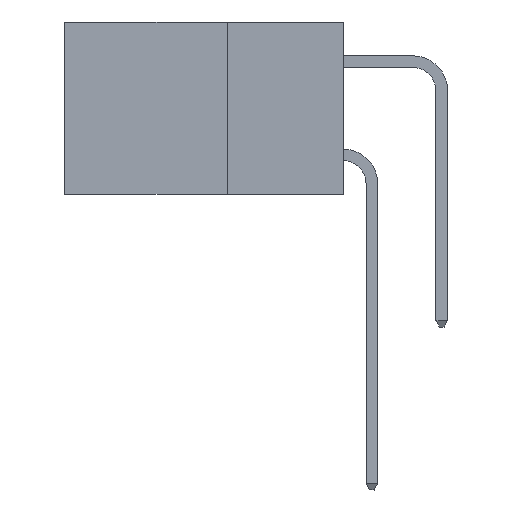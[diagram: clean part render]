
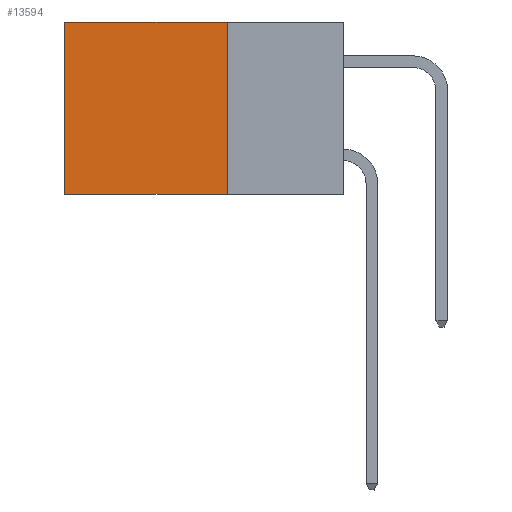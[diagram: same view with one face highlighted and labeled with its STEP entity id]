
A CAD part, left-side view. The second image highlights one B-rep face of the part: STEP entity #13594.
In plain terms, the highlighted planar face has unit normal (-1, 0, 0).
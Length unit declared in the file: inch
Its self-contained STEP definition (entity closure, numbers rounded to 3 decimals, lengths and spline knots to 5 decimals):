
#36 = FACE_OUTER_BOUND ( 'NONE', #26546, .T. ) ;
#1107 = CARTESIAN_POINT ( 'NONE',  ( 0.2615, 0.25, -0.37 ) ) ;
#1275 = VERTEX_POINT ( 'NONE', #7890 ) ;
#1845 = CARTESIAN_POINT ( 'NONE',  ( 0.2615, 0.6, -0.37 ) ) ;
#2565 = VERTEX_POINT ( 'NONE', #1845 ) ;
#5506 = EDGE_CURVE ( 'NONE', #6950, #2565, #26149, .T. ) ;
#5919 = VECTOR ( 'NONE', #23302, 39.37008 ) ;
#6950 = VERTEX_POINT ( 'NONE', #26496 ) ;
#7890 = CARTESIAN_POINT ( 'NONE',  ( 0.2615, 0.25, -0.37 ) ) ;
#8405 = DIRECTION ( 'NONE',  ( 1., 0., 0. ) ) ;
#8439 = AXIS2_PLACEMENT_3D ( 'NONE', #26760, #8405, #14266 ) ;
#8864 = VECTOR ( 'NONE', #10783, 39.37008 ) ;
#9328 = EDGE_CURVE ( 'NONE', #1275, #2565, #17778, .T. ) ;
#9985 = VECTOR ( 'NONE', #20021, 39.37008 ) ;
#10051 = ORIENTED_EDGE ( 'NONE', *, *, #9328, .F. ) ;
#10783 = DIRECTION ( 'NONE',  ( 0., 0., -1. ) ) ;
#12700 = ORIENTED_EDGE ( 'NONE', *, *, #5506, .T. ) ;
#13594 = ADVANCED_FACE ( 'NONE', ( #36 ), #20892, .F. ) ;
#13707 = DIRECTION ( 'NONE',  ( 0., 1., 0. ) ) ;
#14266 = DIRECTION ( 'NONE',  ( 0., 0., -1. ) ) ;
#15179 = ORIENTED_EDGE ( 'NONE', *, *, #17032, .T. ) ;
#16241 = CARTESIAN_POINT ( 'NONE',  ( 0.2615, 0.6, -0.37 ) ) ;
#17032 = EDGE_CURVE ( 'NONE', #18635, #6950, #23548, .T. ) ;
#17778 = LINE ( 'NONE', #1107, #25265 ) ;
#18635 = VERTEX_POINT ( 'NONE', #22100 ) ;
#20021 = DIRECTION ( 'NONE',  ( 0., 0., -1. ) ) ;
#20892 = PLANE ( 'NONE',  #8439 ) ;
#22100 = CARTESIAN_POINT ( 'NONE',  ( 0.2615, 0.25, 0. ) ) ;
#22631 = ORIENTED_EDGE ( 'NONE', *, *, #25621, .F. ) ;
#23164 = CARTESIAN_POINT ( 'NONE',  ( 0.2615, 0.25, 0. ) ) ;
#23287 = LINE ( 'NONE', #24920, #8864 ) ;
#23302 = DIRECTION ( 'NONE',  ( 0., 1., 0. ) ) ;
#23548 = LINE ( 'NONE', #23164, #5919 ) ;
#24920 = CARTESIAN_POINT ( 'NONE',  ( 0.2615, 0.25, -0.37 ) ) ;
#25265 = VECTOR ( 'NONE', #13707, 39.37008 ) ;
#25621 = EDGE_CURVE ( 'NONE', #18635, #1275, #23287, .T. ) ;
#26149 = LINE ( 'NONE', #16241, #9985 ) ;
#26496 = CARTESIAN_POINT ( 'NONE',  ( 0.2615, 0.6, 0. ) ) ;
#26546 = EDGE_LOOP ( 'NONE', ( #12700, #10051, #22631, #15179 ) ) ;
#26760 = CARTESIAN_POINT ( 'NONE',  ( 0.2615, 0.25, -0.37 ) ) ;
